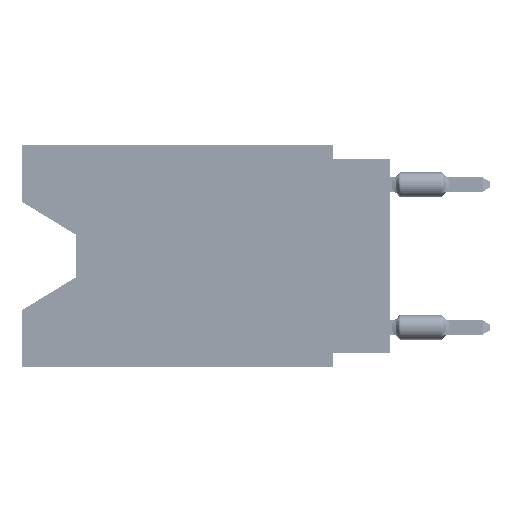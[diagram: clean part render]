
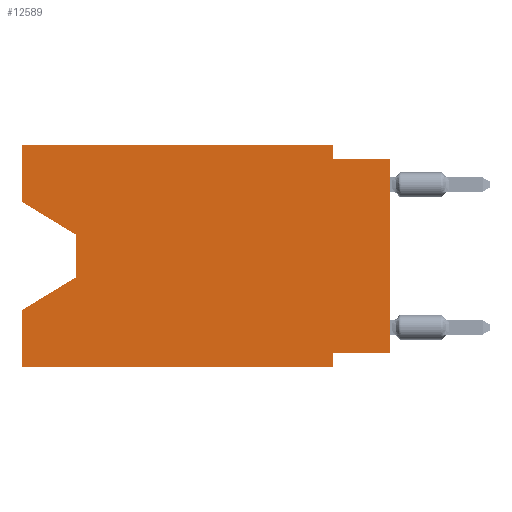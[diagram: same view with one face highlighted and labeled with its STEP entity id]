
A CAD part, left-side view. The second image highlights one B-rep face of the part: STEP entity #12589.
In plain terms, the highlighted planar face has unit normal (-1, 0, 0).
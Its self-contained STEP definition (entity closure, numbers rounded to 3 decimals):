
#238 = PLANE ( 'NONE',  #34010 ) ;
#260 = DIRECTION ( 'NONE',  ( 0., 0., -1. ) ) ;
#408 = ORIENTED_EDGE ( 'NONE', *, *, #37028, .F. ) ;
#517 = EDGE_CURVE ( 'NONE', #9980, #17924, #17866, .T. ) ;
#700 = LINE ( 'NONE', #22660, #44161 ) ;
#884 = LINE ( 'NONE', #37875, #18144 ) ;
#1685 = VERTEX_POINT ( 'NONE', #30898 ) ;
#2068 = DIRECTION ( 'NONE',  ( 0., 0.855, -0.519 ) ) ;
#4334 = VECTOR ( 'NONE', #36227, 1000. ) ;
#4566 = LINE ( 'NONE', #50556, #40495 ) ;
#4672 = DIRECTION ( 'NONE',  ( 0., -1., 0. ) ) ;
#4853 = DIRECTION ( 'NONE',  ( 0., 0., -1. ) ) ;
#5347 = CARTESIAN_POINT ( 'NONE',  ( 0., 2.54, -9.906 ) ) ;
#5384 = DIRECTION ( 'NONE',  ( 0., 0., 1. ) ) ;
#6248 = CARTESIAN_POINT ( 'NONE',  ( 0., 16.383, -2.546 ) ) ;
#6555 = CARTESIAN_POINT ( 'NONE',  ( 0., 2.54, 0. ) ) ;
#6955 = CARTESIAN_POINT ( 'NONE',  ( 0., 2.54, -0.635 ) ) ;
#7683 = EDGE_CURVE ( 'NONE', #38459, #1685, #700, .T. ) ;
#7786 = ORIENTED_EDGE ( 'NONE', *, *, #10142, .T. ) ;
#8215 = DIRECTION ( 'NONE',  ( 0., 0., 1. ) ) ;
#8355 = DIRECTION ( 'NONE',  ( 0., -1., 0. ) ) ;
#8532 = EDGE_LOOP ( 'NONE', ( #58953, #10966, #54465, #57608, #7786, #58603, #48864, #19981, #12889, #408, #13492, #47523 ) ) ;
#9372 = DIRECTION ( 'NONE',  ( 0., 0., 1. ) ) ;
#9464 = EDGE_CURVE ( 'NONE', #17924, #44453, #4566, .T. ) ;
#9608 = LINE ( 'NONE', #46586, #16516 ) ;
#9840 = FACE_OUTER_BOUND ( 'NONE', #8532, .T. ) ;
#9980 = VERTEX_POINT ( 'NONE', #6248 ) ;
#10142 = EDGE_CURVE ( 'NONE', #12529, #43455, #54347, .T. ) ;
#10417 = CARTESIAN_POINT ( 'NONE',  ( 0., 0., -9.271 ) ) ;
#10966 = ORIENTED_EDGE ( 'NONE', *, *, #9464, .T. ) ;
#12529 = VERTEX_POINT ( 'NONE', #57685 ) ;
#12589 = ADVANCED_FACE ( 'NONE', ( #9840 ), #238, .F. ) ;
#12889 = ORIENTED_EDGE ( 'NONE', *, *, #32212, .F. ) ;
#13148 = CARTESIAN_POINT ( 'NONE',  ( 0., 2.54, -9.906 ) ) ;
#13492 = ORIENTED_EDGE ( 'NONE', *, *, #59352, .F. ) ;
#13735 = CARTESIAN_POINT ( 'NONE',  ( 0., 16.383, -9.906 ) ) ;
#13927 = DIRECTION ( 'NONE',  ( 0., 1., 0. ) ) ;
#14021 = VECTOR ( 'NONE', #8215, 1000. ) ;
#16516 = VECTOR ( 'NONE', #5384, 1000. ) ;
#17866 = LINE ( 'NONE', #31706, #4334 ) ;
#17924 = VERTEX_POINT ( 'NONE', #28921 ) ;
#18144 = VECTOR ( 'NONE', #2068, 1000. ) ;
#18292 = LINE ( 'NONE', #5347, #27881 ) ;
#19981 = ORIENTED_EDGE ( 'NONE', *, *, #44250, .T. ) ;
#20793 = EDGE_CURVE ( 'NONE', #9980, #49824, #54496, .T. ) ;
#21584 = CARTESIAN_POINT ( 'NONE',  ( 0., 0., -0.635 ) ) ;
#21787 = VECTOR ( 'NONE', #4672, 1000. ) ;
#22660 = CARTESIAN_POINT ( 'NONE',  ( 0., 0., -9.271 ) ) ;
#23731 = CARTESIAN_POINT ( 'NONE',  ( 0., 2.54, 0. ) ) ;
#26843 = LINE ( 'NONE', #35885, #14021 ) ;
#27881 = VECTOR ( 'NONE', #260, 1000. ) ;
#28921 = CARTESIAN_POINT ( 'NONE',  ( 0., 13.97, -4.013 ) ) ;
#29421 = VECTOR ( 'NONE', #9372, 1000. ) ;
#29988 = EDGE_CURVE ( 'NONE', #44453, #53887, #884, .T. ) ;
#30054 = VERTEX_POINT ( 'NONE', #23731 ) ;
#30898 = CARTESIAN_POINT ( 'NONE',  ( 0., 2.54, -9.271 ) ) ;
#31706 = CARTESIAN_POINT ( 'NONE',  ( 0., 16.383, -2.546 ) ) ;
#32212 = EDGE_CURVE ( 'NONE', #45657, #34191, #35733, .T. ) ;
#33207 = EDGE_CURVE ( 'NONE', #12529, #53887, #9608, .T. ) ;
#34010 = AXIS2_PLACEMENT_3D ( 'NONE', #50455, #36631, #36931 ) ;
#34191 = VERTEX_POINT ( 'NONE', #52131 ) ;
#35733 = LINE ( 'NONE', #21584, #44362 ) ;
#35885 = CARTESIAN_POINT ( 'NONE',  ( 0., 0., 0. ) ) ;
#36227 = DIRECTION ( 'NONE',  ( 0., -0.855, -0.519 ) ) ;
#36631 = DIRECTION ( 'NONE',  ( 1., 0., 0. ) ) ;
#36931 = DIRECTION ( 'NONE',  ( 0., 0., -1. ) ) ;
#37028 = EDGE_CURVE ( 'NONE', #30054, #45657, #52853, .T. ) ;
#37875 = CARTESIAN_POINT ( 'NONE',  ( 0., 13.97, -5.893 ) ) ;
#38459 = VERTEX_POINT ( 'NONE', #10417 ) ;
#40495 = VECTOR ( 'NONE', #4853, 1000. ) ;
#41383 = CARTESIAN_POINT ( 'NONE',  ( 0., 16.383, 0. ) ) ;
#43455 = VERTEX_POINT ( 'NONE', #13148 ) ;
#43852 = DIRECTION ( 'NONE',  ( 0., 0., -1. ) ) ;
#44161 = VECTOR ( 'NONE', #13927, 1000. ) ;
#44250 = EDGE_CURVE ( 'NONE', #38459, #34191, #26843, .T. ) ;
#44362 = VECTOR ( 'NONE', #8355, 1000. ) ;
#44453 = VERTEX_POINT ( 'NONE', #56843 ) ;
#44574 = VECTOR ( 'NONE', #43852, 1000. ) ;
#45657 = VERTEX_POINT ( 'NONE', #6955 ) ;
#46586 = CARTESIAN_POINT ( 'NONE',  ( 0., 16.383, 0. ) ) ;
#47523 = ORIENTED_EDGE ( 'NONE', *, *, #20793, .F. ) ;
#48864 = ORIENTED_EDGE ( 'NONE', *, *, #7683, .F. ) ;
#49824 = VERTEX_POINT ( 'NONE', #53837 ) ;
#50455 = CARTESIAN_POINT ( 'NONE',  ( 0., 16.383, 0. ) ) ;
#50556 = CARTESIAN_POINT ( 'NONE',  ( 0., 13.97, -4.013 ) ) ;
#50726 = EDGE_CURVE ( 'NONE', #1685, #43455, #18292, .T. ) ;
#50957 = VECTOR ( 'NONE', #54644, 1000. ) ;
#51235 = CARTESIAN_POINT ( 'NONE',  ( 0., 16.383, -7.36 ) ) ;
#52131 = CARTESIAN_POINT ( 'NONE',  ( 0., 0., -0.635 ) ) ;
#52853 = LINE ( 'NONE', #6555, #44574 ) ;
#53837 = CARTESIAN_POINT ( 'NONE',  ( 0., 16.383, 0. ) ) ;
#53887 = VERTEX_POINT ( 'NONE', #51235 ) ;
#54347 = LINE ( 'NONE', #13735, #50957 ) ;
#54465 = ORIENTED_EDGE ( 'NONE', *, *, #29988, .T. ) ;
#54496 = LINE ( 'NONE', #55367, #29421 ) ;
#54644 = DIRECTION ( 'NONE',  ( 0., -1., 0. ) ) ;
#55367 = CARTESIAN_POINT ( 'NONE',  ( 0., 16.383, 0. ) ) ;
#56843 = CARTESIAN_POINT ( 'NONE',  ( 0., 13.97, -5.893 ) ) ;
#57608 = ORIENTED_EDGE ( 'NONE', *, *, #33207, .F. ) ;
#57685 = CARTESIAN_POINT ( 'NONE',  ( 0., 16.383, -9.906 ) ) ;
#58603 = ORIENTED_EDGE ( 'NONE', *, *, #50726, .F. ) ;
#58953 = ORIENTED_EDGE ( 'NONE', *, *, #517, .T. ) ;
#59101 = LINE ( 'NONE', #41383, #21787 ) ;
#59352 = EDGE_CURVE ( 'NONE', #49824, #30054, #59101, .T. ) ;
